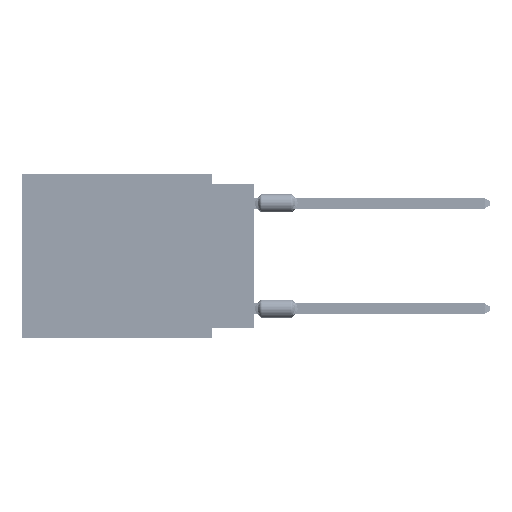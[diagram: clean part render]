
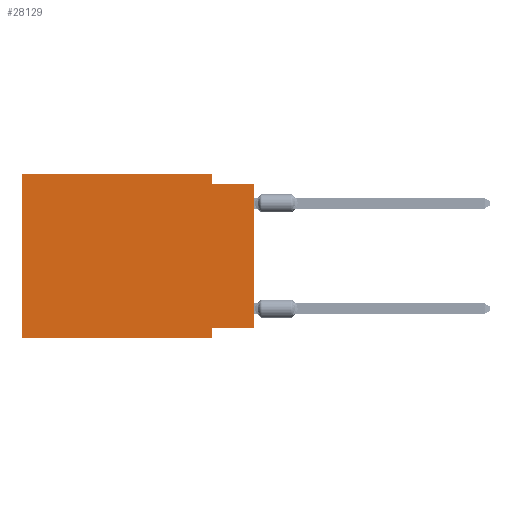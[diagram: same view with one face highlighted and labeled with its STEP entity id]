
A CAD part, left-side view. The second image highlights one B-rep face of the part: STEP entity #28129.
In plain terms, the highlighted planar face has unit normal (-1, 0, 0).
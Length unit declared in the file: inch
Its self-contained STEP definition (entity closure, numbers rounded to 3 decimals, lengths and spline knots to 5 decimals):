
#3309 = VECTOR ( 'NONE', #22413, 39.37008 ) ;
#4637 = LINE ( 'NONE', #72428, #34420 ) ;
#5122 = VECTOR ( 'NONE', #14394, 39.37008 ) ;
#6997 = VERTEX_POINT ( 'NONE', #30370 ) ;
#12000 = ORIENTED_EDGE ( 'NONE', *, *, #14012, .F. ) ;
#13734 = VECTOR ( 'NONE', #73348, 39.37008 ) ;
#13836 = CARTESIAN_POINT ( 'NONE',  ( 0., 0.55, -0.39 ) ) ;
#14012 = EDGE_CURVE ( 'NONE', #32198, #33242, #64618, .T. ) ;
#14394 = DIRECTION ( 'NONE',  ( 0., -1., 0. ) ) ;
#16557 = DIRECTION ( 'NONE',  ( 1., 0., 0. ) ) ;
#16851 = LINE ( 'NONE', #34001, #3309 ) ;
#17013 = DIRECTION ( 'NONE',  ( 0., 1., 0. ) ) ;
#17503 = LINE ( 'NONE', #53434, #77561 ) ;
#18214 = VERTEX_POINT ( 'NONE', #13836 ) ;
#18890 = VERTEX_POINT ( 'NONE', #41976 ) ;
#19685 = LINE ( 'NONE', #62359, #64012 ) ;
#19879 = AXIS2_PLACEMENT_3D ( 'NONE', #41251, #16557, #60787 ) ;
#20399 = VECTOR ( 'NONE', #30585, 39.37008 ) ;
#20758 = CARTESIAN_POINT ( 'NONE',  ( 0., 0., -0.025 ) ) ;
#21315 = VECTOR ( 'NONE', #34827, 39.37008 ) ;
#22413 = DIRECTION ( 'NONE',  ( 0., -1., 0. ) ) ;
#23919 = LINE ( 'NONE', #54228, #13734 ) ;
#26046 = EDGE_CURVE ( 'NONE', #6997, #31037, #17503, .T. ) ;
#27099 = ORIENTED_EDGE ( 'NONE', *, *, #58016, .F. ) ;
#28129 = ADVANCED_FACE ( 'NONE', ( #42432 ), #36453, .F. ) ;
#29377 = ORIENTED_EDGE ( 'NONE', *, *, #51499, .T. ) ;
#29736 = EDGE_CURVE ( 'NONE', #33242, #39272, #77485, .T. ) ;
#30370 = CARTESIAN_POINT ( 'NONE',  ( 0., 0.1, -0.365 ) ) ;
#30585 = DIRECTION ( 'NONE',  ( 0., -1., 0. ) ) ;
#31037 = VERTEX_POINT ( 'NONE', #77105 ) ;
#32159 = ORIENTED_EDGE ( 'NONE', *, *, #29736, .F. ) ;
#32198 = VERTEX_POINT ( 'NONE', #49749 ) ;
#33242 = VERTEX_POINT ( 'NONE', #60959 ) ;
#34001 = CARTESIAN_POINT ( 'NONE',  ( 0., 0.55, -0.39 ) ) ;
#34420 = VECTOR ( 'NONE', #17013, 39.37008 ) ;
#34827 = DIRECTION ( 'NONE',  ( 0., 0., -1. ) ) ;
#36453 = PLANE ( 'NONE',  #19879 ) ;
#39272 = VERTEX_POINT ( 'NONE', #49534 ) ;
#40381 = ORIENTED_EDGE ( 'NONE', *, *, #60587, .F. ) ;
#40786 = CARTESIAN_POINT ( 'NONE',  ( 0., 0.1, 0. ) ) ;
#41251 = CARTESIAN_POINT ( 'NONE',  ( 0., 0.55, 0. ) ) ;
#41654 = EDGE_CURVE ( 'NONE', #18890, #6997, #4637, .T. ) ;
#41976 = CARTESIAN_POINT ( 'NONE',  ( 0., 0., -0.365 ) ) ;
#42432 = FACE_OUTER_BOUND ( 'NONE', #47863, .T. ) ;
#42490 = ORIENTED_EDGE ( 'NONE', *, *, #53144, .T. ) ;
#42516 = CARTESIAN_POINT ( 'NONE',  ( 0., 0.55, 0. ) ) ;
#46948 = CARTESIAN_POINT ( 'NONE',  ( 0., 0., -0.025 ) ) ;
#47863 = EDGE_LOOP ( 'NONE', ( #42490, #27099, #32159, #12000, #40381, #29377, #57188, #53132 ) ) ;
#49534 = CARTESIAN_POINT ( 'NONE',  ( 0., 0.1, -0.025 ) ) ;
#49749 = CARTESIAN_POINT ( 'NONE',  ( 0., 0.55, 0. ) ) ;
#51499 = EDGE_CURVE ( 'NONE', #18214, #31037, #16851, .T. ) ;
#52386 = VERTEX_POINT ( 'NONE', #46948 ) ;
#53132 = ORIENTED_EDGE ( 'NONE', *, *, #41654, .F. ) ;
#53144 = EDGE_CURVE ( 'NONE', #18890, #52386, #23919, .T. ) ;
#53434 = CARTESIAN_POINT ( 'NONE',  ( 0., 0.1, -0.39 ) ) ;
#54228 = CARTESIAN_POINT ( 'NONE',  ( 0., 0., 0. ) ) ;
#57188 = ORIENTED_EDGE ( 'NONE', *, *, #26046, .F. ) ;
#58016 = EDGE_CURVE ( 'NONE', #39272, #52386, #68631, .T. ) ;
#60587 = EDGE_CURVE ( 'NONE', #18214, #32198, #19685, .T. ) ;
#60787 = DIRECTION ( 'NONE',  ( 0., 0., -1. ) ) ;
#60959 = CARTESIAN_POINT ( 'NONE',  ( 0., 0.1, 0. ) ) ;
#62359 = CARTESIAN_POINT ( 'NONE',  ( 0., 0.55, 0. ) ) ;
#64012 = VECTOR ( 'NONE', #69932, 39.37008 ) ;
#64618 = LINE ( 'NONE', #42516, #20399 ) ;
#65403 = DIRECTION ( 'NONE',  ( 0., 0., -1. ) ) ;
#68631 = LINE ( 'NONE', #20758, #5122 ) ;
#69932 = DIRECTION ( 'NONE',  ( 0., 0., 1. ) ) ;
#72428 = CARTESIAN_POINT ( 'NONE',  ( 0., 0., -0.365 ) ) ;
#73348 = DIRECTION ( 'NONE',  ( 0., 0., 1. ) ) ;
#77105 = CARTESIAN_POINT ( 'NONE',  ( 0., 0.1, -0.39 ) ) ;
#77485 = LINE ( 'NONE', #40786, #21315 ) ;
#77561 = VECTOR ( 'NONE', #65403, 39.37008 ) ;
